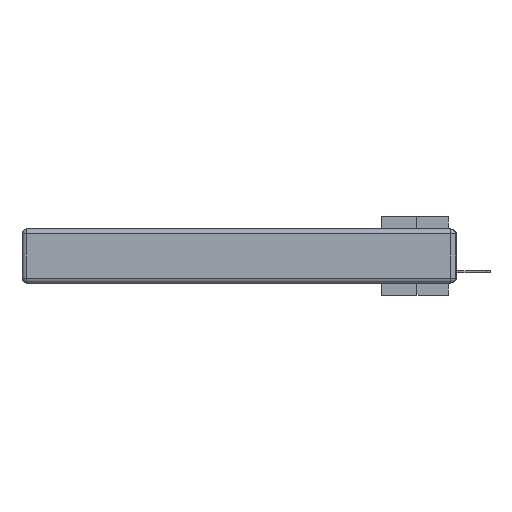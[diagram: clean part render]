
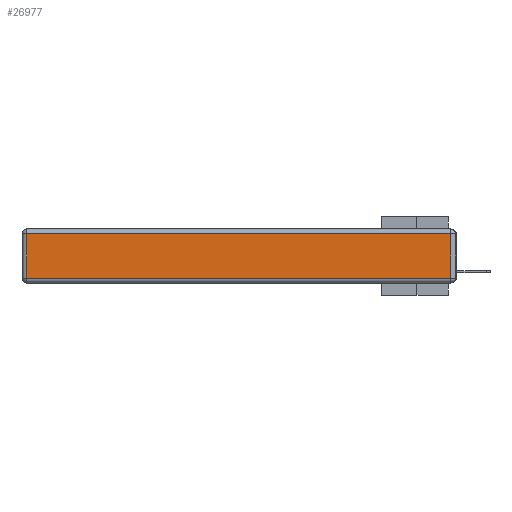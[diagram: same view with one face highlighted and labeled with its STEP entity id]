
A CAD part, left-side view. The second image highlights one B-rep face of the part: STEP entity #26977.
In plain terms, the highlighted planar face has unit normal (-1, 0, 0).
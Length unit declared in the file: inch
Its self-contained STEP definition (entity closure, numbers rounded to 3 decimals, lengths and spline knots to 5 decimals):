
#539 = CARTESIAN_POINT ( 'NONE',  ( 0., 2.72, -0.343 ) ) ;
#769 = CARTESIAN_POINT ( 'NONE',  ( 0., 0., -0.313 ) ) ;
#891 = DIRECTION ( 'NONE',  ( 0., 0., 1. ) ) ;
#1197 = FACE_OUTER_BOUND ( 'NONE', #13092, .T. ) ;
#1385 = ORIENTED_EDGE ( 'NONE', *, *, #27255, .T. ) ;
#2615 = VECTOR ( 'NONE', #28839, 39.37008 ) ;
#3852 = VERTEX_POINT ( 'NONE', #7202 ) ;
#4237 = VECTOR ( 'NONE', #29313, 39.37008 ) ;
#5172 = ORIENTED_EDGE ( 'NONE', *, *, #6773, .T. ) ;
#6015 = CARTESIAN_POINT ( 'NONE',  ( 0., 0., -0.343 ) ) ;
#6383 = VERTEX_POINT ( 'NONE', #26914 ) ;
#6773 = EDGE_CURVE ( 'NONE', #14036, #3852, #29232, .T. ) ;
#7202 = CARTESIAN_POINT ( 'NONE',  ( 0., 2.72, -0.313 ) ) ;
#12069 = DIRECTION ( 'NONE',  ( 0., 0., 1. ) ) ;
#13092 = EDGE_LOOP ( 'NONE', ( #21406, #1385, #26368, #5172 ) ) ;
#14036 = VERTEX_POINT ( 'NONE', #18535 ) ;
#15529 = LINE ( 'NONE', #769, #4237 ) ;
#17499 = VERTEX_POINT ( 'NONE', #24694 ) ;
#17845 = EDGE_CURVE ( 'NONE', #17499, #14036, #23292, .T. ) ;
#17977 = DIRECTION ( 'NONE',  ( -1., 0., 0. ) ) ;
#18298 = VECTOR ( 'NONE', #19804, 39.37008 ) ;
#18400 = VECTOR ( 'NONE', #12069, 39.37008 ) ;
#18535 = CARTESIAN_POINT ( 'NONE',  ( 0., 2.72, -0.03 ) ) ;
#19804 = DIRECTION ( 'NONE',  ( 0., 0., -1. ) ) ;
#20047 = EDGE_CURVE ( 'NONE', #3852, #6383, #15529, .T. ) ;
#21383 = CARTESIAN_POINT ( 'NONE',  ( 0., 0.03, -0.343 ) ) ;
#21406 = ORIENTED_EDGE ( 'NONE', *, *, #20047, .T. ) ;
#21838 = LINE ( 'NONE', #21383, #18400 ) ;
#23292 = LINE ( 'NONE', #30571, #2615 ) ;
#24694 = CARTESIAN_POINT ( 'NONE',  ( 0., 0.03, -0.03 ) ) ;
#24815 = AXIS2_PLACEMENT_3D ( 'NONE', #6015, #17977, #891 ) ;
#26368 = ORIENTED_EDGE ( 'NONE', *, *, #17845, .T. ) ;
#26914 = CARTESIAN_POINT ( 'NONE',  ( 0., 0.03, -0.313 ) ) ;
#26977 = ADVANCED_FACE ( 'NONE', ( #1197 ), #27117, .T. ) ;
#27117 = PLANE ( 'NONE',  #24815 ) ;
#27255 = EDGE_CURVE ( 'NONE', #6383, #17499, #21838, .T. ) ;
#28839 = DIRECTION ( 'NONE',  ( 0., 1., 0. ) ) ;
#29232 = LINE ( 'NONE', #539, #18298 ) ;
#29313 = DIRECTION ( 'NONE',  ( 0., -1., 0. ) ) ;
#30571 = CARTESIAN_POINT ( 'NONE',  ( 0., 2.75, -0.03 ) ) ;
